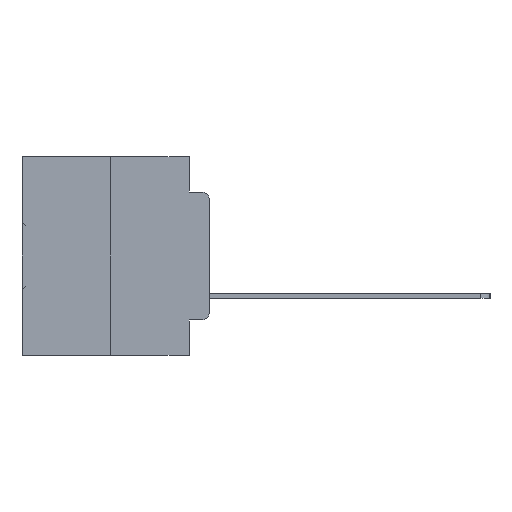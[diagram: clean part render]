
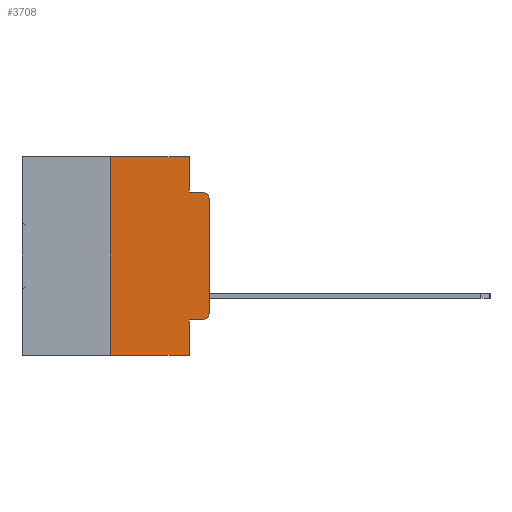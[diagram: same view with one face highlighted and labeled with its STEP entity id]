
A CAD part, left-side view. The second image highlights one B-rep face of the part: STEP entity #3708.
In plain terms, the highlighted planar face has unit normal (-1, 0, 0).
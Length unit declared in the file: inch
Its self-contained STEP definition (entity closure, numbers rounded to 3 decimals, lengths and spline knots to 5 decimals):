
#328 = CIRCLE ( 'NONE', #6642, 0.02 ) ;
#428 = AXIS2_PLACEMENT_3D ( 'NONE', #22894, #9656, #22810 ) ;
#513 = CARTESIAN_POINT ( 'NONE',  ( 0., 0.051, 0. ) ) ;
#942 = VERTEX_POINT ( 'NONE', #17172 ) ;
#1052 = EDGE_CURVE ( 'NONE', #31192, #1761, #10179, .T. ) ;
#1277 = ORIENTED_EDGE ( 'NONE', *, *, #10145, .F. ) ;
#1322 = DIRECTION ( 'NONE',  ( 0., -1., 0. ) ) ;
#1361 = VERTEX_POINT ( 'NONE', #6706 ) ;
#1621 = VECTOR ( 'NONE', #1322, 39.37008 ) ;
#1659 = CARTESIAN_POINT ( 'NONE',  ( 0., 0.02, -0.0885 ) ) ;
#1723 = DIRECTION ( 'NONE',  ( 0., -1., 0. ) ) ;
#1761 = VERTEX_POINT ( 'NONE', #2410 ) ;
#1763 = CARTESIAN_POINT ( 'NONE',  ( 0., 0.051, -0.4115 ) ) ;
#2202 = EDGE_CURVE ( 'NONE', #942, #1361, #5447, .T. ) ;
#2410 = CARTESIAN_POINT ( 'NONE',  ( 0., 0., -0.1085 ) ) ;
#2670 = LINE ( 'NONE', #513, #16874 ) ;
#2966 = VECTOR ( 'NONE', #23911, 39.37008 ) ;
#3380 = VERTEX_POINT ( 'NONE', #25126 ) ;
#3696 = VERTEX_POINT ( 'NONE', #1659 ) ;
#3708 = ADVANCED_FACE ( 'NONE', ( #14159 ), #25506, .F. ) ;
#5447 = LINE ( 'NONE', #1763, #12578 ) ;
#5537 = ORIENTED_EDGE ( 'NONE', *, *, #2202, .T. ) ;
#5549 = CIRCLE ( 'NONE', #17588, 0.02 ) ;
#6642 = AXIS2_PLACEMENT_3D ( 'NONE', #9753, #27986, #12430 ) ;
#6706 = CARTESIAN_POINT ( 'NONE',  ( 0., 0.02, -0.4115 ) ) ;
#8329 = EDGE_CURVE ( 'NONE', #1761, #3696, #328, .T. ) ;
#8913 = CARTESIAN_POINT ( 'NONE',  ( 0., 0.051, 0. ) ) ;
#9572 = LINE ( 'NONE', #30592, #15785 ) ;
#9656 = DIRECTION ( 'NONE',  ( 1., 0., 0. ) ) ;
#9753 = CARTESIAN_POINT ( 'NONE',  ( 0., 0.02, -0.1085 ) ) ;
#9760 = CARTESIAN_POINT ( 'NONE',  ( 0., 0.051, -0.0885 ) ) ;
#10000 = VERTEX_POINT ( 'NONE', #17131 ) ;
#10145 = EDGE_CURVE ( 'NONE', #11493, #3696, #19735, .T. ) ;
#10179 = LINE ( 'NONE', #16704, #2966 ) ;
#10196 = ORIENTED_EDGE ( 'NONE', *, *, #22529, .F. ) ;
#11027 = ORIENTED_EDGE ( 'NONE', *, *, #22375, .F. ) ;
#11493 = VERTEX_POINT ( 'NONE', #29149 ) ;
#12430 = DIRECTION ( 'NONE',  ( 0., 0., -1. ) ) ;
#12522 = DIRECTION ( 'NONE',  ( 0., 0., 1. ) ) ;
#12578 = VECTOR ( 'NONE', #1723, 39.37008 ) ;
#12671 = ORIENTED_EDGE ( 'NONE', *, *, #25224, .T. ) ;
#13608 = CARTESIAN_POINT ( 'NONE',  ( 0., 0., -0.3915 ) ) ;
#14159 = FACE_OUTER_BOUND ( 'NONE', #21835, .T. ) ;
#14323 = DIRECTION ( 'NONE',  ( -1., 0., 0. ) ) ;
#15442 = EDGE_CURVE ( 'NONE', #19684, #11493, #18596, .T. ) ;
#15736 = CARTESIAN_POINT ( 'NONE',  ( 0., 0.473, 0. ) ) ;
#15785 = VECTOR ( 'NONE', #12522, 39.37008 ) ;
#15896 = VERTEX_POINT ( 'NONE', #32023 ) ;
#16704 = CARTESIAN_POINT ( 'NONE',  ( 0., 0., 0. ) ) ;
#16874 = VECTOR ( 'NONE', #19146, 39.37008 ) ;
#16884 = DIRECTION ( 'NONE',  ( 0., 0., -1. ) ) ;
#17131 = CARTESIAN_POINT ( 'NONE',  ( 0., 0.25, -0.5 ) ) ;
#17172 = CARTESIAN_POINT ( 'NONE',  ( 0., 0.051, -0.4115 ) ) ;
#17315 = CARTESIAN_POINT ( 'NONE',  ( 0., 0.473, -0.5 ) ) ;
#17588 = AXIS2_PLACEMENT_3D ( 'NONE', #29805, #14323, #32345 ) ;
#17792 = VECTOR ( 'NONE', #16884, 39.37008 ) ;
#17973 = ORIENTED_EDGE ( 'NONE', *, *, #20393, .T. ) ;
#18596 = LINE ( 'NONE', #8913, #17792 ) ;
#18938 = VECTOR ( 'NONE', #25406, 39.37008 ) ;
#19146 = DIRECTION ( 'NONE',  ( 0., 0., -1. ) ) ;
#19684 = VERTEX_POINT ( 'NONE', #31852 ) ;
#19735 = LINE ( 'NONE', #9760, #18938 ) ;
#19975 = ORIENTED_EDGE ( 'NONE', *, *, #1052, .T. ) ;
#20393 = EDGE_CURVE ( 'NONE', #10000, #15896, #28011, .T. ) ;
#21835 = EDGE_LOOP ( 'NONE', ( #19975, #26902, #1277, #23266, #10196, #11027, #17973, #25697, #5537, #12671 ) ) ;
#22375 = EDGE_CURVE ( 'NONE', #10000, #3380, #9572, .T. ) ;
#22529 = EDGE_CURVE ( 'NONE', #3380, #19684, #30673, .T. ) ;
#22810 = DIRECTION ( 'NONE',  ( 0., 0., -1. ) ) ;
#22894 = CARTESIAN_POINT ( 'NONE',  ( 0., 0.473, 0. ) ) ;
#23266 = ORIENTED_EDGE ( 'NONE', *, *, #15442, .F. ) ;
#23911 = DIRECTION ( 'NONE',  ( 0., 0., 1. ) ) ;
#24700 = VECTOR ( 'NONE', #26049, 39.37008 ) ;
#25126 = CARTESIAN_POINT ( 'NONE',  ( 0., 0.25, 0. ) ) ;
#25224 = EDGE_CURVE ( 'NONE', #1361, #31192, #5549, .T. ) ;
#25406 = DIRECTION ( 'NONE',  ( 0., -1., 0. ) ) ;
#25506 = PLANE ( 'NONE',  #428 ) ;
#25697 = ORIENTED_EDGE ( 'NONE', *, *, #29297, .F. ) ;
#26049 = DIRECTION ( 'NONE',  ( 0., -1., 0. ) ) ;
#26902 = ORIENTED_EDGE ( 'NONE', *, *, #8329, .T. ) ;
#27986 = DIRECTION ( 'NONE',  ( -1., 0., 0. ) ) ;
#28011 = LINE ( 'NONE', #17315, #1621 ) ;
#29149 = CARTESIAN_POINT ( 'NONE',  ( 0., 0.051, -0.0885 ) ) ;
#29297 = EDGE_CURVE ( 'NONE', #942, #15896, #2670, .T. ) ;
#29805 = CARTESIAN_POINT ( 'NONE',  ( 0., 0.02, -0.3915 ) ) ;
#30592 = CARTESIAN_POINT ( 'NONE',  ( 0., 0.25, 0. ) ) ;
#30673 = LINE ( 'NONE', #15736, #24700 ) ;
#31192 = VERTEX_POINT ( 'NONE', #13608 ) ;
#31852 = CARTESIAN_POINT ( 'NONE',  ( 0., 0.051, 0. ) ) ;
#32023 = CARTESIAN_POINT ( 'NONE',  ( 0., 0.051, -0.5 ) ) ;
#32345 = DIRECTION ( 'NONE',  ( 0., 0., -1. ) ) ;
